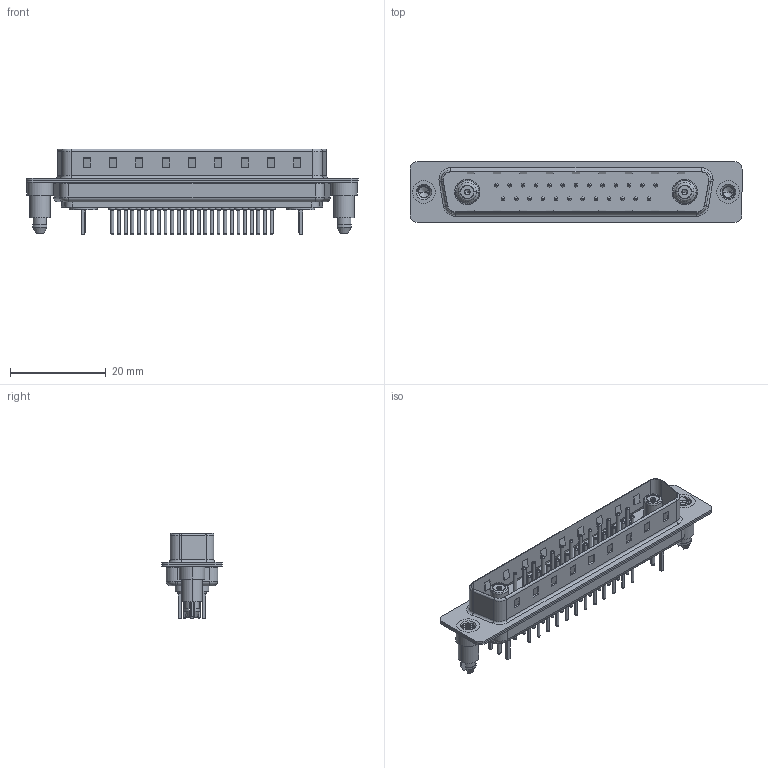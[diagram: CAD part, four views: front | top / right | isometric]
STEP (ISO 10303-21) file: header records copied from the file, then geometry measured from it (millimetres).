
FILE_DESCRIPTION (( 'STEP AP203' ), '1' );
FILE_NAME ('627-27W2224-7TD.STEP', '2019-05-30T03:50:18', ( '' ), ( '' ), 'SwSTEP 2.0', 'SolidWorks 2016', '' );
FILE_SCHEMA (( 'CONFIG_CONTROL_DESIGN' ));
Length unit declared in the file: millimetre
Products named in the file (14): Socket_Str; 627Combo Housing_27W2; Co-Ax Jack Assy_S; 627Combo Shell Rear_37 Contacts; 627Combo Threaded Boardlock_5; 627Combo Shell Front_37 Contacts; 627Combo Contact Row 1_24; 627Combo Threaded Boardlock_D; 627Combo Contact Row 2_24; Co-Ax Jack_Straight PC Tail; 627-27W2224-7TD; Insulator Socket; Insulator Socket 2; Locking Collar
Assembly tree (37 placements, depth 3):
  627-27W2224-7TD
    627Combo Housing_27W2
    627Combo Shell Rear_37 Contacts
    627Combo Shell Front_37 Contacts
    627Combo Threaded Boardlock_D
    Co-Ax Jack Assy_S  x2
      Co-Ax Jack_Straight PC Tail
      Insulator Socket
      Insulator Socket 2
      Locking Collar
      Socket_Str
    627Combo Threaded Boardlock_5
    627Combo Contact Row 1_24  x13
    627Combo Contact Row 2_24  x12
Bounding box: 69.3 x 12.6 x 17.9 mm (x, y, z)
Volume: 3936.4 mm3; surface area: 10202.8 mm2
Topology: 40 solids, 40 shells, 1617 faces, 3557 edges, 2176 vertices
Faces by surface type: cylinder 625, plane 488, torus 458, cone 31, bspline 11, sphere 4
Entity records: 30793 total; most frequent: CARTESIAN_POINT 8323, DIRECTION 4496, ORIENTED_EDGE 4044, EDGE_CURVE 2022, AXIS2_PLACEMENT_3D 1747, VERTEX_POINT 1292, EDGE_LOOP 1042, VECTOR 1002
